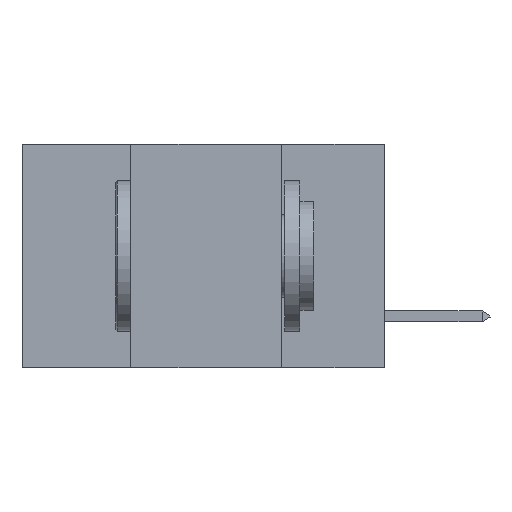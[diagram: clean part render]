
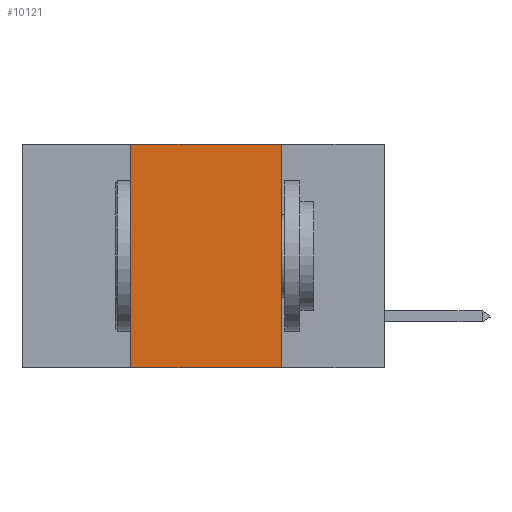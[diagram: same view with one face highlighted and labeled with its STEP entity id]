
A CAD part, left-side view. The second image highlights one B-rep face of the part: STEP entity #10121.
In plain terms, the highlighted planar face has unit normal (-1, 0, 0).
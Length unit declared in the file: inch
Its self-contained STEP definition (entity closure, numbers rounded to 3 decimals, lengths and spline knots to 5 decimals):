
#1025 = VECTOR ( 'NONE', #12268, 39.37008 ) ;
#3466 = VECTOR ( 'NONE', #17785, 39.37008 ) ;
#4520 = LINE ( 'NONE', #34752, #3466 ) ;
#4643 = ORIENTED_EDGE ( 'NONE', *, *, #12859, .F. ) ;
#6532 = EDGE_CURVE ( 'NONE', #30436, #38745, #24213, .T. ) ;
#7735 = EDGE_CURVE ( 'NONE', #30436, #30411, #32558, .T. ) ;
#9585 = VECTOR ( 'NONE', #38492, 39.37008 ) ;
#10121 = ADVANCED_FACE ( 'NONE', ( #32302 ), #41674, .F. ) ;
#11337 = CARTESIAN_POINT ( 'NONE',  ( 0., 0.17, 0. ) ) ;
#11963 = ORIENTED_EDGE ( 'NONE', *, *, #6532, .F. ) ;
#12268 = DIRECTION ( 'NONE',  ( 0., 0., 1. ) ) ;
#12859 = EDGE_CURVE ( 'NONE', #29506, #30411, #40190, .T. ) ;
#14676 = DIRECTION ( 'NONE',  ( 0., 0., -1. ) ) ;
#15808 = EDGE_LOOP ( 'NONE', ( #4643, #18996, #11963, #31148 ) ) ;
#16094 = AXIS2_PLACEMENT_3D ( 'NONE', #18371, #38278, #14676 ) ;
#17785 = DIRECTION ( 'NONE',  ( 0., -1., 0. ) ) ;
#18371 = CARTESIAN_POINT ( 'NONE',  ( 0., 0.6, 0. ) ) ;
#18996 = ORIENTED_EDGE ( 'NONE', *, *, #28403, .F. ) ;
#24213 = LINE ( 'NONE', #39401, #1025 ) ;
#24487 = CARTESIAN_POINT ( 'NONE',  ( 0., 0.42, -0.37 ) ) ;
#28166 = CARTESIAN_POINT ( 'NONE',  ( 0., 0.17, -0.37 ) ) ;
#28403 = EDGE_CURVE ( 'NONE', #38745, #29506, #4520, .T. ) ;
#28851 = CARTESIAN_POINT ( 'NONE',  ( 0., 0.42, 0. ) ) ;
#29506 = VERTEX_POINT ( 'NONE', #30040 ) ;
#30040 = CARTESIAN_POINT ( 'NONE',  ( 0., 0.17, 0. ) ) ;
#30411 = VERTEX_POINT ( 'NONE', #28166 ) ;
#30436 = VERTEX_POINT ( 'NONE', #24487 ) ;
#31148 = ORIENTED_EDGE ( 'NONE', *, *, #7735, .T. ) ;
#32302 = FACE_OUTER_BOUND ( 'NONE', #15808, .T. ) ;
#32558 = LINE ( 'NONE', #38875, #36259 ) ;
#34752 = CARTESIAN_POINT ( 'NONE',  ( 0., 0.6, 0. ) ) ;
#36259 = VECTOR ( 'NONE', #39067, 39.37008 ) ;
#38278 = DIRECTION ( 'NONE',  ( 1., 0., 0. ) ) ;
#38492 = DIRECTION ( 'NONE',  ( 0., 0., -1. ) ) ;
#38745 = VERTEX_POINT ( 'NONE', #28851 ) ;
#38875 = CARTESIAN_POINT ( 'NONE',  ( 0., 0.6, -0.37 ) ) ;
#39067 = DIRECTION ( 'NONE',  ( 0., -1., 0. ) ) ;
#39401 = CARTESIAN_POINT ( 'NONE',  ( 0., 0.42, 0. ) ) ;
#40190 = LINE ( 'NONE', #11337, #9585 ) ;
#41674 = PLANE ( 'NONE',  #16094 ) ;
